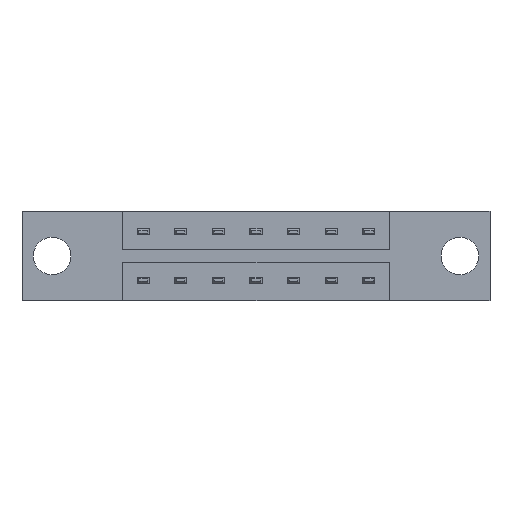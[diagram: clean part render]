
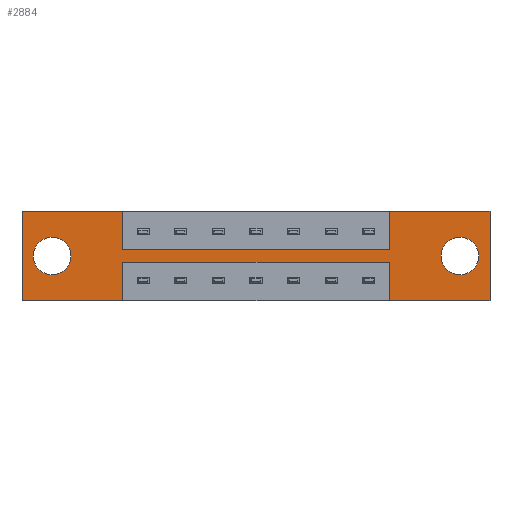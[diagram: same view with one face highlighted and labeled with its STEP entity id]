
A CAD part, front view. The second image highlights one B-rep face of the part: STEP entity #2884.
In plain terms, the highlighted planar face has unit normal (0, -1, 0).
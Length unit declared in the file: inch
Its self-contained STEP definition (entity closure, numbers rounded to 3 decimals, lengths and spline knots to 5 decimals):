
#8 = AXIS2_PLACEMENT_3D ( 'NONE', #8173, #8093, #8082 ) ;
#55 = CARTESIAN_POINT ( 'NONE',  ( 0., 0., -0.37 ) ) ;
#246 = VERTEX_POINT ( 'NONE', #6364 ) ;
#289 = DIRECTION ( 'NONE',  ( 0., 0., 1. ) ) ;
#357 = VECTOR ( 'NONE', #6436, 39.37008 ) ;
#434 = LINE ( 'NONE', #4835, #7537 ) ;
#517 = DIRECTION ( 'NONE',  ( 0., 0., 1. ) ) ;
#723 = DIRECTION ( 'NONE',  ( 0., 1., 0. ) ) ;
#730 = CARTESIAN_POINT ( 'NONE',  ( 0.125, 0., -0.185 ) ) ;
#797 = CARTESIAN_POINT ( 'NONE',  ( 1.5225, 0., -0.2115 ) ) ;
#878 = CARTESIAN_POINT ( 'NONE',  ( 0.4175, 0., -0.2115 ) ) ;
#909 = DIRECTION ( 'NONE',  ( 0., 0., 1. ) ) ;
#949 = DIRECTION ( 'NONE',  ( -1., 0., 0. ) ) ;
#1003 = EDGE_CURVE ( 'NONE', #3157, #5301, #3090, .T. ) ;
#1090 = LINE ( 'NONE', #3250, #6299 ) ;
#1095 = ORIENTED_EDGE ( 'NONE', *, *, #2483, .F. ) ;
#1159 = ORIENTED_EDGE ( 'NONE', *, *, #1003, .T. ) ;
#1201 = EDGE_CURVE ( 'NONE', #8180, #246, #6691, .T. ) ;
#1375 = ORIENTED_EDGE ( 'NONE', *, *, #1992, .T. ) ;
#1489 = CARTESIAN_POINT ( 'NONE',  ( 1.94, 0., 0. ) ) ;
#1525 = ORIENTED_EDGE ( 'NONE', *, *, #4307, .T. ) ;
#1563 = VERTEX_POINT ( 'NONE', #6482 ) ;
#1643 = LINE ( 'NONE', #8434, #1882 ) ;
#1658 = CARTESIAN_POINT ( 'NONE',  ( 1.5225, 0., -0.2115 ) ) ;
#1669 = VECTOR ( 'NONE', #949, 39.37008 ) ;
#1695 = VECTOR ( 'NONE', #6116, 39.37008 ) ;
#1882 = VECTOR ( 'NONE', #3180, 39.37008 ) ;
#1928 = CARTESIAN_POINT ( 'NONE',  ( 0.4175, 0., -0.37 ) ) ;
#1992 = EDGE_CURVE ( 'NONE', #246, #8180, #2758, .T. ) ;
#2056 = FACE_OUTER_BOUND ( 'NONE', #4957, .T. ) ;
#2068 = ORIENTED_EDGE ( 'NONE', *, *, #4627, .F. ) ;
#2157 = CARTESIAN_POINT ( 'NONE',  ( 1.815, 0., -0.185 ) ) ;
#2240 = ORIENTED_EDGE ( 'NONE', *, *, #3046, .F. ) ;
#2357 = VECTOR ( 'NONE', #517, 39.37008 ) ;
#2483 = EDGE_CURVE ( 'NONE', #6387, #8439, #8834, .T. ) ;
#2615 = EDGE_LOOP ( 'NONE', ( #1375, #3169 ) ) ;
#2694 = VERTEX_POINT ( 'NONE', #3477 ) ;
#2758 = CIRCLE ( 'NONE', #4382, 0.078 ) ;
#2876 = DIRECTION ( 'NONE',  ( 0., 0., -1. ) ) ;
#2884 = ADVANCED_FACE ( 'NONE', ( #5443, #3927, #2056 ), #8102, .T. ) ;
#2891 = ORIENTED_EDGE ( 'NONE', *, *, #5713, .F. ) ;
#2893 = CARTESIAN_POINT ( 'NONE',  ( 0., 0., 0. ) ) ;
#2920 = ORIENTED_EDGE ( 'NONE', *, *, #7516, .F. ) ;
#3046 = EDGE_CURVE ( 'NONE', #2694, #5148, #5953, .T. ) ;
#3076 = ORIENTED_EDGE ( 'NONE', *, *, #4249, .F. ) ;
#3090 = CIRCLE ( 'NONE', #8503, 0.078 ) ;
#3106 = EDGE_CURVE ( 'NONE', #1563, #3629, #3808, .T. ) ;
#3157 = VERTEX_POINT ( 'NONE', #5453 ) ;
#3169 = ORIENTED_EDGE ( 'NONE', *, *, #1201, .T. ) ;
#3180 = DIRECTION ( 'NONE',  ( -1., 0., 0. ) ) ;
#3228 = DIRECTION ( 'NONE',  ( 0., 1., 0. ) ) ;
#3250 = CARTESIAN_POINT ( 'NONE',  ( 0.4175, 0., -0.1585 ) ) ;
#3336 = CARTESIAN_POINT ( 'NONE',  ( 1.5225, 0., -0.37 ) ) ;
#3344 = VECTOR ( 'NONE', #6066, 39.37008 ) ;
#3477 = CARTESIAN_POINT ( 'NONE',  ( 0., 0., -0.37 ) ) ;
#3564 = CARTESIAN_POINT ( 'NONE',  ( 0.125, 0., -0.263 ) ) ;
#3565 = LINE ( 'NONE', #55, #1669 ) ;
#3629 = VERTEX_POINT ( 'NONE', #1489 ) ;
#3751 = ORIENTED_EDGE ( 'NONE', *, *, #8419, .F. ) ;
#3807 = ORIENTED_EDGE ( 'NONE', *, *, #7377, .F. ) ;
#3808 = LINE ( 'NONE', #6135, #1695 ) ;
#3847 = ORIENTED_EDGE ( 'NONE', *, *, #8119, .F. ) ;
#3927 = FACE_BOUND ( 'NONE', #2615, .T. ) ;
#3952 = CARTESIAN_POINT ( 'NONE',  ( 0.4175, 0., -0.1585 ) ) ;
#3974 = VECTOR ( 'NONE', #5069, 39.37008 ) ;
#4069 = ORIENTED_EDGE ( 'NONE', *, *, #6209, .F. ) ;
#4155 = CARTESIAN_POINT ( 'NONE',  ( 0.4175, 0., -0.1585 ) ) ;
#4249 = EDGE_CURVE ( 'NONE', #7176, #4782, #7780, .T. ) ;
#4307 = EDGE_CURVE ( 'NONE', #5301, #3157, #7365, .T. ) ;
#4380 = LINE ( 'NONE', #8611, #2357 ) ;
#4382 = AXIS2_PLACEMENT_3D ( 'NONE', #730, #723, #289 ) ;
#4533 = CARTESIAN_POINT ( 'NONE',  ( 1.815, 0., -0.185 ) ) ;
#4584 = CARTESIAN_POINT ( 'NONE',  ( 0.4175, 0., 0. ) ) ;
#4622 = ORIENTED_EDGE ( 'NONE', *, *, #7813, .F. ) ;
#4627 = EDGE_CURVE ( 'NONE', #8309, #6387, #3565, .T. ) ;
#4703 = CARTESIAN_POINT ( 'NONE',  ( 0.125, 0., -0.185 ) ) ;
#4704 = VECTOR ( 'NONE', #4809, 39.37008 ) ;
#4762 = CARTESIAN_POINT ( 'NONE',  ( 0.4175, 0., -0.2115 ) ) ;
#4782 = VERTEX_POINT ( 'NONE', #3952 ) ;
#4809 = DIRECTION ( 'NONE',  ( 0., 0., -1. ) ) ;
#4835 = CARTESIAN_POINT ( 'NONE',  ( 0.4175, 0., -0.2115 ) ) ;
#4879 = DIRECTION ( 'NONE',  ( 1., 0., 0. ) ) ;
#4957 = EDGE_LOOP ( 'NONE', ( #1095, #2068, #2891, #7445, #3807, #4622, #3076, #2920, #2240, #4069, #3847, #3751 ) ) ;
#5069 = DIRECTION ( 'NONE',  ( -1., 0., 0. ) ) ;
#5148 = VERTEX_POINT ( 'NONE', #2893 ) ;
#5246 = DIRECTION ( 'NONE',  ( 1., 0., 0. ) ) ;
#5299 = DIRECTION ( 'NONE',  ( 0., 0., 1. ) ) ;
#5301 = VERTEX_POINT ( 'NONE', #8343 ) ;
#5308 = LINE ( 'NONE', #8602, #3344 ) ;
#5443 = FACE_BOUND ( 'NONE', #7009, .T. ) ;
#5450 = VECTOR ( 'NONE', #909, 39.37008 ) ;
#5453 = CARTESIAN_POINT ( 'NONE',  ( 1.815, 0., -0.107 ) ) ;
#5487 = DIRECTION ( 'NONE',  ( 0., 0., -1. ) ) ;
#5488 = LINE ( 'NONE', #878, #3974 ) ;
#5504 = LINE ( 'NONE', #8121, #6411 ) ;
#5713 = EDGE_CURVE ( 'NONE', #3629, #8309, #5308, .T. ) ;
#5953 = LINE ( 'NONE', #6398, #357 ) ;
#5959 = CARTESIAN_POINT ( 'NONE',  ( 1.5225, 0., -0.1585 ) ) ;
#6066 = DIRECTION ( 'NONE',  ( 0., 0., -1. ) ) ;
#6116 = DIRECTION ( 'NONE',  ( 1., 0., 0. ) ) ;
#6135 = CARTESIAN_POINT ( 'NONE',  ( 0., 0., 0. ) ) ;
#6209 = EDGE_CURVE ( 'NONE', #7915, #2694, #1643, .T. ) ;
#6294 = AXIS2_PLACEMENT_3D ( 'NONE', #2157, #6835, #2876 ) ;
#6299 = VECTOR ( 'NONE', #5246, 39.37008 ) ;
#6364 = CARTESIAN_POINT ( 'NONE',  ( 0.125, 0., -0.107 ) ) ;
#6387 = VERTEX_POINT ( 'NONE', #3336 ) ;
#6398 = CARTESIAN_POINT ( 'NONE',  ( 0., 0., 0. ) ) ;
#6411 = VECTOR ( 'NONE', #4879, 39.37008 ) ;
#6436 = DIRECTION ( 'NONE',  ( 0., 0., 1. ) ) ;
#6482 = CARTESIAN_POINT ( 'NONE',  ( 1.5225, 0., 0. ) ) ;
#6691 = CIRCLE ( 'NONE', #7939, 0.078 ) ;
#6835 = DIRECTION ( 'NONE',  ( 0., 1., 0. ) ) ;
#7009 = EDGE_LOOP ( 'NONE', ( #1159, #1525 ) ) ;
#7176 = VERTEX_POINT ( 'NONE', #4584 ) ;
#7270 = VERTEX_POINT ( 'NONE', #5959 ) ;
#7365 = CIRCLE ( 'NONE', #6294, 0.078 ) ;
#7377 = EDGE_CURVE ( 'NONE', #7270, #1563, #4380, .T. ) ;
#7382 = VERTEX_POINT ( 'NONE', #4762 ) ;
#7445 = ORIENTED_EDGE ( 'NONE', *, *, #3106, .F. ) ;
#7516 = EDGE_CURVE ( 'NONE', #5148, #7176, #5504, .T. ) ;
#7537 = VECTOR ( 'NONE', #5487, 39.37008 ) ;
#7569 = CARTESIAN_POINT ( 'NONE',  ( 1.94, 0., -0.37 ) ) ;
#7757 = DIRECTION ( 'NONE',  ( 0., 1., 0. ) ) ;
#7780 = LINE ( 'NONE', #4155, #4704 ) ;
#7813 = EDGE_CURVE ( 'NONE', #4782, #7270, #1090, .T. ) ;
#7915 = VERTEX_POINT ( 'NONE', #1928 ) ;
#7939 = AXIS2_PLACEMENT_3D ( 'NONE', #4703, #3228, #5299 ) ;
#8082 = DIRECTION ( 'NONE',  ( 0., 0., -1. ) ) ;
#8093 = DIRECTION ( 'NONE',  ( 0., -1., 0. ) ) ;
#8102 = PLANE ( 'NONE',  #8 ) ;
#8119 = EDGE_CURVE ( 'NONE', #7382, #7915, #434, .T. ) ;
#8121 = CARTESIAN_POINT ( 'NONE',  ( 0., 0., 0. ) ) ;
#8173 = CARTESIAN_POINT ( 'NONE',  ( 0., 0., -0.37 ) ) ;
#8180 = VERTEX_POINT ( 'NONE', #3564 ) ;
#8298 = DIRECTION ( 'NONE',  ( 0., 0., -1. ) ) ;
#8309 = VERTEX_POINT ( 'NONE', #7569 ) ;
#8343 = CARTESIAN_POINT ( 'NONE',  ( 1.815, 0., -0.263 ) ) ;
#8419 = EDGE_CURVE ( 'NONE', #8439, #7382, #5488, .T. ) ;
#8434 = CARTESIAN_POINT ( 'NONE',  ( 0., 0., -0.37 ) ) ;
#8439 = VERTEX_POINT ( 'NONE', #1658 ) ;
#8503 = AXIS2_PLACEMENT_3D ( 'NONE', #4533, #7757, #8298 ) ;
#8602 = CARTESIAN_POINT ( 'NONE',  ( 1.94, 0., 0. ) ) ;
#8611 = CARTESIAN_POINT ( 'NONE',  ( 1.5225, 0., -0.1585 ) ) ;
#8834 = LINE ( 'NONE', #797, #5450 ) ;
